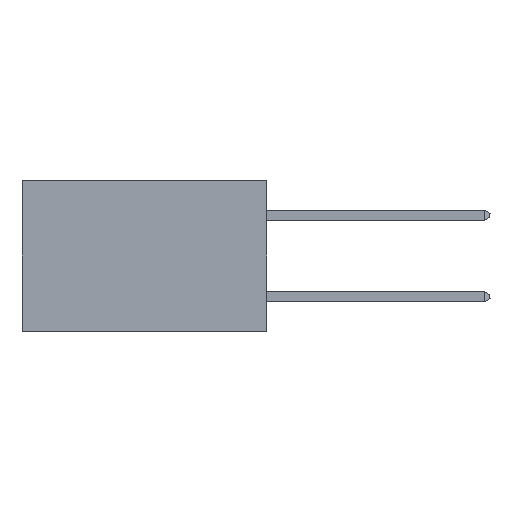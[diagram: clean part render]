
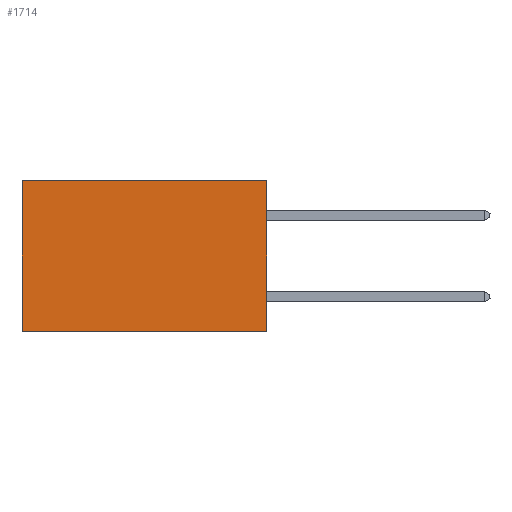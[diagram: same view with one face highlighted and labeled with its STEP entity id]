
A CAD part, left-side view. The second image highlights one B-rep face of the part: STEP entity #1714.
In plain terms, the highlighted planar face has unit normal (-1, 0, 0).
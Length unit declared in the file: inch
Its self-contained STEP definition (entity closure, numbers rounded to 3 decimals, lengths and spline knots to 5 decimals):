
#155 = CARTESIAN_POINT ( 'NONE',  ( 0.2875, 0.6, 0. ) ) ;
#528 = PLANE ( 'NONE',  #32388 ) ;
#540 = DIRECTION ( 'NONE',  ( 0., 0., -1. ) ) ;
#1714 = ADVANCED_FACE ( 'NONE', ( #28611 ), #528, .F. ) ;
#3991 = CARTESIAN_POINT ( 'NONE',  ( 0.2875, 0., 0. ) ) ;
#4054 = VECTOR ( 'NONE', #23006, 39.37008 ) ;
#6499 = EDGE_CURVE ( 'NONE', #39181, #28088, #22598, .T. ) ;
#6836 = DIRECTION ( 'NONE',  ( 1., 0., 0. ) ) ;
#7902 = LINE ( 'NONE', #37913, #12748 ) ;
#10732 = LINE ( 'NONE', #3991, #34295 ) ;
#12370 = ORIENTED_EDGE ( 'NONE', *, *, #23029, .F. ) ;
#12748 = VECTOR ( 'NONE', #19985, 39.37008 ) ;
#12905 = CARTESIAN_POINT ( 'NONE',  ( 0.2875, 0., 0. ) ) ;
#13998 = CARTESIAN_POINT ( 'NONE',  ( 0.2875, 0., -0.37 ) ) ;
#14180 = LINE ( 'NONE', #13998, #4054 ) ;
#14519 = CARTESIAN_POINT ( 'NONE',  ( 0.2875, 0., -0.37 ) ) ;
#19985 = DIRECTION ( 'NONE',  ( 0., 0., -1. ) ) ;
#20082 = ORIENTED_EDGE ( 'NONE', *, *, #38735, .T. ) ;
#20124 = CARTESIAN_POINT ( 'NONE',  ( 0.2875, 0.6, -0.37 ) ) ;
#21507 = VERTEX_POINT ( 'NONE', #20124 ) ;
#22598 = LINE ( 'NONE', #25014, #37043 ) ;
#23006 = DIRECTION ( 'NONE',  ( 0., 1., 0. ) ) ;
#23029 = EDGE_CURVE ( 'NONE', #28088, #21507, #14180, .T. ) ;
#23494 = EDGE_CURVE ( 'NONE', #39181, #37325, #10732, .T. ) ;
#24361 = ORIENTED_EDGE ( 'NONE', *, *, #6499, .F. ) ;
#25014 = CARTESIAN_POINT ( 'NONE',  ( 0.2875, 0., 0. ) ) ;
#25759 = DIRECTION ( 'NONE',  ( 0., 1., 0. ) ) ;
#26720 = EDGE_LOOP ( 'NONE', ( #20082, #12370, #24361, #29947 ) ) ;
#28088 = VERTEX_POINT ( 'NONE', #14519 ) ;
#28375 = DIRECTION ( 'NONE',  ( 0., 0., -1. ) ) ;
#28611 = FACE_OUTER_BOUND ( 'NONE', #26720, .T. ) ;
#29947 = ORIENTED_EDGE ( 'NONE', *, *, #23494, .T. ) ;
#32388 = AXIS2_PLACEMENT_3D ( 'NONE', #12905, #6836, #28375 ) ;
#34295 = VECTOR ( 'NONE', #25759, 39.37008 ) ;
#37043 = VECTOR ( 'NONE', #540, 39.37008 ) ;
#37179 = CARTESIAN_POINT ( 'NONE',  ( 0.2875, 0., 0. ) ) ;
#37325 = VERTEX_POINT ( 'NONE', #155 ) ;
#37913 = CARTESIAN_POINT ( 'NONE',  ( 0.2875, 0.6, 0. ) ) ;
#38735 = EDGE_CURVE ( 'NONE', #37325, #21507, #7902, .T. ) ;
#39181 = VERTEX_POINT ( 'NONE', #37179 ) ;
